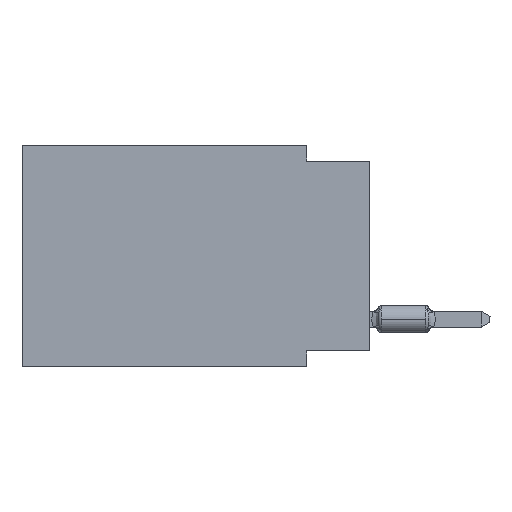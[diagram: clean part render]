
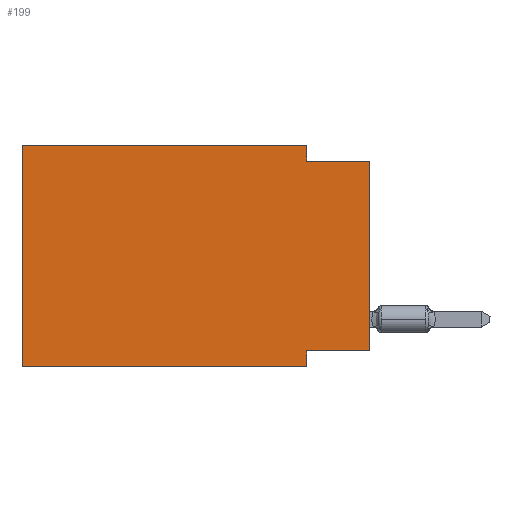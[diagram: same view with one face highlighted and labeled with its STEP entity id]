
A CAD part, left-side view. The second image highlights one B-rep face of the part: STEP entity #199.
In plain terms, the highlighted planar face has unit normal (-1, 0, 0).
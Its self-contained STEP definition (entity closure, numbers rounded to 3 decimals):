
#199 = ADVANCED_FACE ( 'NONE', ( #287 ), #32098, .F. ) ;
#287 = FACE_OUTER_BOUND ( 'NONE', #24268, .T. ) ;
#296 = EDGE_CURVE ( 'NONE', #5499, #42422, #34178, .T. ) ;
#375 = VECTOR ( 'NONE', #20628, 1000. ) ;
#1317 = ORIENTED_EDGE ( 'NONE', *, *, #21494, .F. ) ;
#1407 = VECTOR ( 'NONE', #41670, 1000. ) ;
#2742 = LINE ( 'NONE', #35717, #33402 ) ;
#3225 = DIRECTION ( 'NONE',  ( 0., -1., 0. ) ) ;
#3608 = ORIENTED_EDGE ( 'NONE', *, *, #22001, .T. ) ;
#5499 = VERTEX_POINT ( 'NONE', #9999 ) ;
#5645 = AXIS2_PLACEMENT_3D ( 'NONE', #11128, #18447, #39879 ) ;
#7181 = CARTESIAN_POINT ( 'NONE',  ( 0., 13.97, -8.89 ) ) ;
#7783 = VECTOR ( 'NONE', #16256, 1000. ) ;
#8949 = CARTESIAN_POINT ( 'NONE',  ( 0., 13.97, 0. ) ) ;
#8982 = CARTESIAN_POINT ( 'NONE',  ( 0., 0., -0.635 ) ) ;
#9979 = VERTEX_POINT ( 'NONE', #28847 ) ;
#9999 = CARTESIAN_POINT ( 'NONE',  ( 0., 2.54, -0.635 ) ) ;
#10260 = ORIENTED_EDGE ( 'NONE', *, *, #17585, .T. ) ;
#10700 = CARTESIAN_POINT ( 'NONE',  ( 0., 0., -8.255 ) ) ;
#10701 = CARTESIAN_POINT ( 'NONE',  ( 0., 0., -8.255 ) ) ;
#11128 = CARTESIAN_POINT ( 'NONE',  ( 0., 13.97, 0. ) ) ;
#13945 = EDGE_CURVE ( 'NONE', #22487, #9979, #35727, .T. ) ;
#14022 = ORIENTED_EDGE ( 'NONE', *, *, #296, .F. ) ;
#16256 = DIRECTION ( 'NONE',  ( 0., 0., -1. ) ) ;
#16625 = CARTESIAN_POINT ( 'NONE',  ( 0., 13.97, -8.89 ) ) ;
#17585 = EDGE_CURVE ( 'NONE', #31878, #46195, #39474, .T. ) ;
#18447 = DIRECTION ( 'NONE',  ( 1., 0., 0. ) ) ;
#18983 = ORIENTED_EDGE ( 'NONE', *, *, #28686, .F. ) ;
#20628 = DIRECTION ( 'NONE',  ( 0., 1., 0. ) ) ;
#20729 = CARTESIAN_POINT ( 'NONE',  ( 0., 2.54, -8.89 ) ) ;
#21494 = EDGE_CURVE ( 'NONE', #28696, #46195, #30861, .T. ) ;
#21596 = DIRECTION ( 'NONE',  ( 0., -1., 0. ) ) ;
#22001 = EDGE_CURVE ( 'NONE', #35926, #42422, #2742, .T. ) ;
#22487 = VERTEX_POINT ( 'NONE', #8949 ) ;
#22849 = LINE ( 'NONE', #26599, #1407 ) ;
#23533 = EDGE_CURVE ( 'NONE', #35926, #28696, #39671, .T. ) ;
#24268 = EDGE_LOOP ( 'NONE', ( #3608, #14022, #37625, #40964, #18983, #10260, #1317, #42239 ) ) ;
#26599 = CARTESIAN_POINT ( 'NONE',  ( 0., 13.97, 0. ) ) ;
#28177 = VECTOR ( 'NONE', #3225, 1000. ) ;
#28686 = EDGE_CURVE ( 'NONE', #31878, #22487, #22849, .T. ) ;
#28696 = VERTEX_POINT ( 'NONE', #34364 ) ;
#28847 = CARTESIAN_POINT ( 'NONE',  ( 0., 2.54, 0. ) ) ;
#30861 = LINE ( 'NONE', #20729, #7783 ) ;
#31187 = DIRECTION ( 'NONE',  ( 0., 0., -1. ) ) ;
#31425 = LINE ( 'NONE', #44698, #32192 ) ;
#31878 = VERTEX_POINT ( 'NONE', #16625 ) ;
#32098 = PLANE ( 'NONE',  #5645 ) ;
#32178 = DIRECTION ( 'NONE',  ( 0., 0., 1. ) ) ;
#32192 = VECTOR ( 'NONE', #31187, 1000. ) ;
#32656 = CARTESIAN_POINT ( 'NONE',  ( 0., 0., -0.635 ) ) ;
#32933 = EDGE_CURVE ( 'NONE', #9979, #5499, #31425, .T. ) ;
#33402 = VECTOR ( 'NONE', #32178, 1000. ) ;
#34178 = LINE ( 'NONE', #8982, #41039 ) ;
#34364 = CARTESIAN_POINT ( 'NONE',  ( 0., 2.54, -8.255 ) ) ;
#35717 = CARTESIAN_POINT ( 'NONE',  ( 0., 0., 0. ) ) ;
#35727 = LINE ( 'NONE', #38802, #28177 ) ;
#35926 = VERTEX_POINT ( 'NONE', #10700 ) ;
#37625 = ORIENTED_EDGE ( 'NONE', *, *, #32933, .F. ) ;
#37910 = CARTESIAN_POINT ( 'NONE',  ( 0., 2.54, -8.89 ) ) ;
#38802 = CARTESIAN_POINT ( 'NONE',  ( 0., 13.97, 0. ) ) ;
#39474 = LINE ( 'NONE', #7181, #40041 ) ;
#39671 = LINE ( 'NONE', #10701, #375 ) ;
#39879 = DIRECTION ( 'NONE',  ( 0., 0., -1. ) ) ;
#40041 = VECTOR ( 'NONE', #21596, 1000. ) ;
#40964 = ORIENTED_EDGE ( 'NONE', *, *, #13945, .F. ) ;
#41039 = VECTOR ( 'NONE', #45038, 1000. ) ;
#41670 = DIRECTION ( 'NONE',  ( 0., 0., 1. ) ) ;
#42239 = ORIENTED_EDGE ( 'NONE', *, *, #23533, .F. ) ;
#42422 = VERTEX_POINT ( 'NONE', #32656 ) ;
#44698 = CARTESIAN_POINT ( 'NONE',  ( 0., 2.54, 0. ) ) ;
#45038 = DIRECTION ( 'NONE',  ( 0., -1., 0. ) ) ;
#46195 = VERTEX_POINT ( 'NONE', #37910 ) ;
